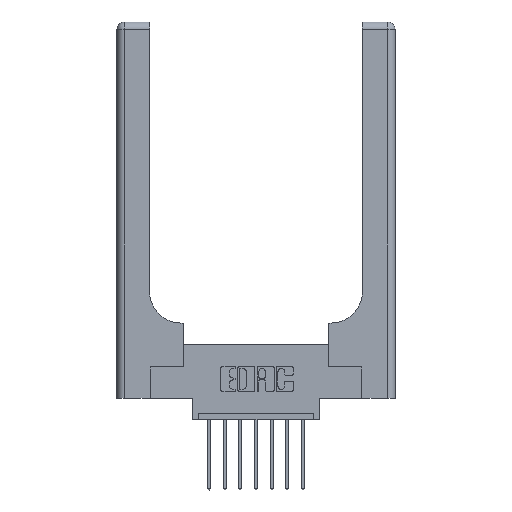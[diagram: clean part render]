
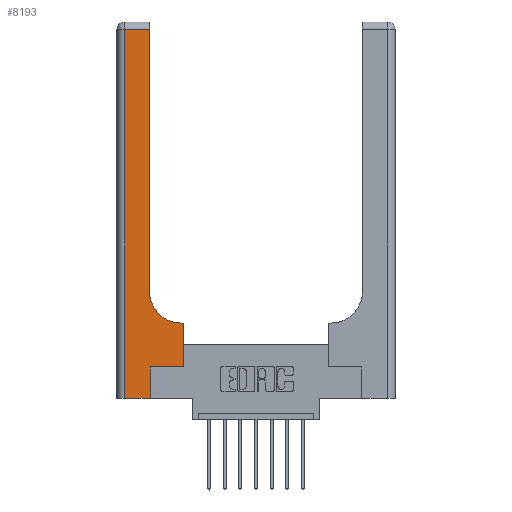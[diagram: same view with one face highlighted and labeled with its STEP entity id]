
A CAD part, top view. The second image highlights one B-rep face of the part: STEP entity #8193.
In plain terms, the highlighted planar face has unit normal (0, 0, 1).
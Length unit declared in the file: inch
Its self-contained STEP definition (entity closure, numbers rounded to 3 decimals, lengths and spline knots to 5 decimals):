
#45 = VERTEX_POINT ( 'NONE', #10476 ) ;
#68 = VERTEX_POINT ( 'NONE', #10581 ) ;
#269 = CARTESIAN_POINT ( 'NONE',  ( 0.51, 0.85, 0.37 ) ) ;
#271 = LINE ( 'NONE', #9740, #5999 ) ;
#424 = LINE ( 'NONE', #11007, #8946 ) ;
#619 = LINE ( 'NONE', #8370, #7220 ) ;
#718 = EDGE_CURVE ( 'NONE', #45, #2963, #13871, .T. ) ;
#920 = ORIENTED_EDGE ( 'NONE', *, *, #5746, .T. ) ;
#939 = CARTESIAN_POINT ( 'NONE',  ( 0.528, 0.25, 0.37 ) ) ;
#1028 = EDGE_CURVE ( 'NONE', #7459, #1045, #9143, .T. ) ;
#1045 = VERTEX_POINT ( 'NONE', #7957 ) ;
#1777 = LINE ( 'NONE', #10050, #8035 ) ;
#1994 = LINE ( 'NONE', #12922, #13984 ) ;
#2223 = CARTESIAN_POINT ( 'NONE',  ( 0., 0., 0.37 ) ) ;
#2445 = VECTOR ( 'NONE', #4935, 39.37008 ) ;
#2963 = VERTEX_POINT ( 'NONE', #14061 ) ;
#3124 = DIRECTION ( 'NONE',  ( -1., 0., 0. ) ) ;
#4070 = EDGE_CURVE ( 'NONE', #9010, #10347, #271, .T. ) ;
#4072 = AXIS2_PLACEMENT_3D ( 'NONE', #269, #4866, #12418 ) ;
#4751 = EDGE_LOOP ( 'NONE', ( #9966, #6785, #920, #9224, #9530, #12788, #6152, #5935, #7578 ) ) ;
#4861 = CARTESIAN_POINT ( 'NONE',  ( 0.06, 0., 0.37 ) ) ;
#4866 = DIRECTION ( 'NONE',  ( 0., 0., -1. ) ) ;
#4876 = CARTESIAN_POINT ( 'NONE',  ( 0.26, 0.6, 0.37 ) ) ;
#4935 = DIRECTION ( 'NONE',  ( -1., 0., 0. ) ) ;
#5199 = CARTESIAN_POINT ( 'NONE',  ( 0.26, 3., 0.37 ) ) ;
#5348 = CARTESIAN_POINT ( 'NONE',  ( 0.528, 0.6, 0.37 ) ) ;
#5746 = EDGE_CURVE ( 'NONE', #12862, #7459, #424, .T. ) ;
#5935 = ORIENTED_EDGE ( 'NONE', *, *, #12721, .T. ) ;
#5999 = VECTOR ( 'NONE', #10425, 39.37008 ) ;
#6040 = EDGE_CURVE ( 'NONE', #2963, #12862, #1994, .T. ) ;
#6068 = DIRECTION ( 'NONE',  ( -1., 0., 0. ) ) ;
#6152 = ORIENTED_EDGE ( 'NONE', *, *, #12298, .T. ) ;
#6341 = VERTEX_POINT ( 'NONE', #5348 ) ;
#6761 = CARTESIAN_POINT ( 'NONE',  ( 0.265, 0.25, 0.37 ) ) ;
#6785 = ORIENTED_EDGE ( 'NONE', *, *, #6040, .T. ) ;
#7220 = VECTOR ( 'NONE', #7231, 39.37008 ) ;
#7231 = DIRECTION ( 'NONE',  ( 0., 1., 0. ) ) ;
#7318 = LINE ( 'NONE', #4876, #2445 ) ;
#7459 = VERTEX_POINT ( 'NONE', #4861 ) ;
#7578 = ORIENTED_EDGE ( 'NONE', *, *, #13957, .T. ) ;
#7782 = DIRECTION ( 'NONE',  ( 0., -1., 0. ) ) ;
#7952 = VECTOR ( 'NONE', #14090, 39.37008 ) ;
#7957 = CARTESIAN_POINT ( 'NONE',  ( 0.265, 0., 0.37 ) ) ;
#8035 = VECTOR ( 'NONE', #12131, 39.37008 ) ;
#8193 = ADVANCED_FACE ( 'NONE', ( #11935 ), #11572, .F. ) ;
#8370 = CARTESIAN_POINT ( 'NONE',  ( 0.265, 0., 0.37 ) ) ;
#8538 = CIRCLE ( 'NONE', #4072, 0.25 ) ;
#8946 = VECTOR ( 'NONE', #7782, 39.37008 ) ;
#9010 = VERTEX_POINT ( 'NONE', #6761 ) ;
#9143 = LINE ( 'NONE', #2223, #14022 ) ;
#9224 = ORIENTED_EDGE ( 'NONE', *, *, #1028, .T. ) ;
#9309 = DIRECTION ( 'NONE',  ( 0., 0., -1. ) ) ;
#9530 = ORIENTED_EDGE ( 'NONE', *, *, #14249, .T. ) ;
#9740 = CARTESIAN_POINT ( 'NONE',  ( 0.265, 0.25, 0.37 ) ) ;
#9937 = CARTESIAN_POINT ( 'NONE',  ( 0.06, 2.94, 0.37 ) ) ;
#9966 = ORIENTED_EDGE ( 'NONE', *, *, #718, .T. ) ;
#10050 = CARTESIAN_POINT ( 'NONE',  ( 0.528, 0.25, 0.37 ) ) ;
#10347 = VERTEX_POINT ( 'NONE', #939 ) ;
#10402 = CARTESIAN_POINT ( 'NONE',  ( 0., 3., 0.37 ) ) ;
#10425 = DIRECTION ( 'NONE',  ( 1., 0., 0. ) ) ;
#10476 = CARTESIAN_POINT ( 'NONE',  ( 0.26, 0.85, 0.37 ) ) ;
#10581 = CARTESIAN_POINT ( 'NONE',  ( 0.51, 0.6, 0.37 ) ) ;
#11007 = CARTESIAN_POINT ( 'NONE',  ( 0.06, 3., 0.37 ) ) ;
#11103 = AXIS2_PLACEMENT_3D ( 'NONE', #10402, #9309, #6068 ) ;
#11572 = PLANE ( 'NONE',  #11103 ) ;
#11935 = FACE_OUTER_BOUND ( 'NONE', #4751, .T. ) ;
#12131 = DIRECTION ( 'NONE',  ( 0., 1., 0. ) ) ;
#12298 = EDGE_CURVE ( 'NONE', #10347, #6341, #1777, .T. ) ;
#12418 = DIRECTION ( 'NONE',  ( 1., 0., 0. ) ) ;
#12721 = EDGE_CURVE ( 'NONE', #6341, #68, #7318, .T. ) ;
#12788 = ORIENTED_EDGE ( 'NONE', *, *, #4070, .T. ) ;
#12862 = VERTEX_POINT ( 'NONE', #9937 ) ;
#12922 = CARTESIAN_POINT ( 'NONE',  ( 0., 2.94, 0.37 ) ) ;
#13263 = DIRECTION ( 'NONE',  ( 1., 0., 0. ) ) ;
#13871 = LINE ( 'NONE', #5199, #7952 ) ;
#13957 = EDGE_CURVE ( 'NONE', #68, #45, #8538, .T. ) ;
#13984 = VECTOR ( 'NONE', #3124, 39.37008 ) ;
#14022 = VECTOR ( 'NONE', #13263, 39.37008 ) ;
#14061 = CARTESIAN_POINT ( 'NONE',  ( 0.26, 2.94, 0.37 ) ) ;
#14090 = DIRECTION ( 'NONE',  ( 0., 1., 0. ) ) ;
#14249 = EDGE_CURVE ( 'NONE', #1045, #9010, #619, .T. ) ;
